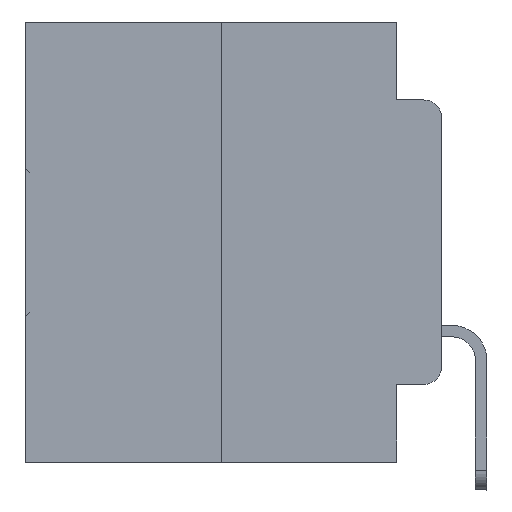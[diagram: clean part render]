
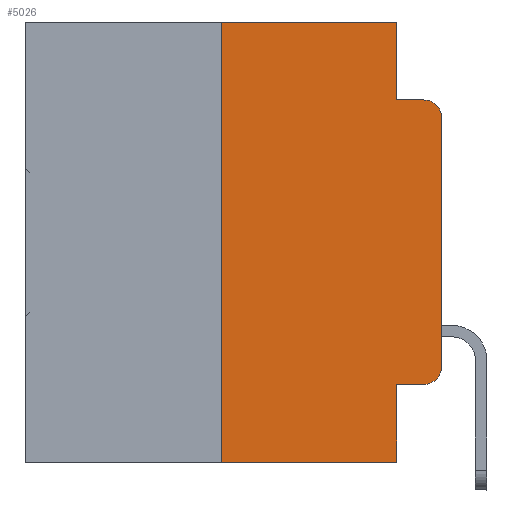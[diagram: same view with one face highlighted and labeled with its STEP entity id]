
A CAD part, left-side view. The second image highlights one B-rep face of the part: STEP entity #5026.
In plain terms, the highlighted planar face has unit normal (-1, 0, 0).
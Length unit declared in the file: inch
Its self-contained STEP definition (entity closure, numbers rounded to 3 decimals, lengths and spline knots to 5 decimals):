
#214 = ORIENTED_EDGE ( 'NONE', *, *, #19649, .F. ) ;
#864 = VERTEX_POINT ( 'NONE', #28707 ) ;
#908 = CARTESIAN_POINT ( 'NONE',  ( 0., 0.473, 0. ) ) ;
#1115 = DIRECTION ( 'NONE',  ( 1., 0., 0. ) ) ;
#1442 = ORIENTED_EDGE ( 'NONE', *, *, #26857, .F. ) ;
#1703 = LINE ( 'NONE', #908, #13015 ) ;
#1744 = DIRECTION ( 'NONE',  ( 0., 0., -1. ) ) ;
#2532 = VERTEX_POINT ( 'NONE', #3071 ) ;
#2735 = ORIENTED_EDGE ( 'NONE', *, *, #4568, .T. ) ;
#2929 = LINE ( 'NONE', #17786, #11492 ) ;
#3071 = CARTESIAN_POINT ( 'NONE',  ( 0., 0., -0.3915 ) ) ;
#3426 = ORIENTED_EDGE ( 'NONE', *, *, #12831, .T. ) ;
#3738 = DIRECTION ( 'NONE',  ( 0., -1., 0. ) ) ;
#3915 = VERTEX_POINT ( 'NONE', #12719 ) ;
#4088 = EDGE_CURVE ( 'NONE', #23201, #19139, #2929, .T. ) ;
#4233 = CARTESIAN_POINT ( 'NONE',  ( 0., 0.02, -0.3915 ) ) ;
#4366 = LINE ( 'NONE', #6525, #6291 ) ;
#4568 = EDGE_CURVE ( 'NONE', #14420, #16784, #14978, .T. ) ;
#4625 = DIRECTION ( 'NONE',  ( 0., 0., 1. ) ) ;
#4961 = EDGE_CURVE ( 'NONE', #18920, #27669, #1703, .T. ) ;
#5026 = ADVANCED_FACE ( 'NONE', ( #26962 ), #18706, .F. ) ;
#5320 = CIRCLE ( 'NONE', #6911, 0.02 ) ;
#5344 = VECTOR ( 'NONE', #4625, 39.37008 ) ;
#5829 = DIRECTION ( 'NONE',  ( 0., 0., -1. ) ) ;
#6291 = VECTOR ( 'NONE', #1744, 39.37008 ) ;
#6369 = AXIS2_PLACEMENT_3D ( 'NONE', #25749, #1115, #18502 ) ;
#6510 = CARTESIAN_POINT ( 'NONE',  ( 0., 0.25, -0.5 ) ) ;
#6525 = CARTESIAN_POINT ( 'NONE',  ( 0., 0.051, 0. ) ) ;
#6529 = CARTESIAN_POINT ( 'NONE',  ( 0., 0.25, 0. ) ) ;
#6729 = DIRECTION ( 'NONE',  ( 0., 0., -1. ) ) ;
#6879 = CARTESIAN_POINT ( 'NONE',  ( 0., 0., 0. ) ) ;
#6911 = AXIS2_PLACEMENT_3D ( 'NONE', #4233, #29305, #6729 ) ;
#6956 = CARTESIAN_POINT ( 'NONE',  ( 0., 0.051, -0.5 ) ) ;
#7088 = ORIENTED_EDGE ( 'NONE', *, *, #9439, .T. ) ;
#7480 = LINE ( 'NONE', #6879, #28429 ) ;
#7897 = VECTOR ( 'NONE', #25131, 39.37008 ) ;
#8065 = CARTESIAN_POINT ( 'NONE',  ( 0., 0.473, -0.5 ) ) ;
#8171 = DIRECTION ( 'NONE',  ( 0., -1., 0. ) ) ;
#8917 = CARTESIAN_POINT ( 'NONE',  ( 0., 0., -0.1085 ) ) ;
#9439 = EDGE_CURVE ( 'NONE', #864, #2532, #5320, .T. ) ;
#9491 = ORIENTED_EDGE ( 'NONE', *, *, #23891, .F. ) ;
#9516 = ORIENTED_EDGE ( 'NONE', *, *, #18030, .T. ) ;
#9901 = ORIENTED_EDGE ( 'NONE', *, *, #23281, .T. ) ;
#11492 = VECTOR ( 'NONE', #5829, 39.37008 ) ;
#11805 = DIRECTION ( 'NONE',  ( 0., 0., 1. ) ) ;
#12719 = CARTESIAN_POINT ( 'NONE',  ( 0., 0.051, -0.0885 ) ) ;
#12831 = EDGE_CURVE ( 'NONE', #27946, #19139, #21442, .T. ) ;
#13015 = VECTOR ( 'NONE', #3738, 39.37008 ) ;
#14321 = DIRECTION ( 'NONE',  ( 0., 0., -1. ) ) ;
#14345 = CARTESIAN_POINT ( 'NONE',  ( 0., 0.051, -0.0885 ) ) ;
#14387 = CARTESIAN_POINT ( 'NONE',  ( 0., 0.051, -0.4115 ) ) ;
#14420 = VERTEX_POINT ( 'NONE', #8917 ) ;
#14978 = CIRCLE ( 'NONE', #28000, 0.02 ) ;
#16452 = ORIENTED_EDGE ( 'NONE', *, *, #4961, .F. ) ;
#16784 = VERTEX_POINT ( 'NONE', #21985 ) ;
#17171 = VECTOR ( 'NONE', #22247, 39.37008 ) ;
#17187 = VECTOR ( 'NONE', #8171, 39.37008 ) ;
#17786 = CARTESIAN_POINT ( 'NONE',  ( 0., 0.051, 0. ) ) ;
#17868 = CARTESIAN_POINT ( 'NONE',  ( 0., 0.051, -0.4115 ) ) ;
#18030 = EDGE_CURVE ( 'NONE', #23201, #864, #28075, .T. ) ;
#18502 = DIRECTION ( 'NONE',  ( 0., 0., -1. ) ) ;
#18706 = PLANE ( 'NONE',  #6369 ) ;
#18715 = ORIENTED_EDGE ( 'NONE', *, *, #4088, .F. ) ;
#18920 = VERTEX_POINT ( 'NONE', #6529 ) ;
#19139 = VERTEX_POINT ( 'NONE', #6956 ) ;
#19496 = CARTESIAN_POINT ( 'NONE',  ( 0., 0.25, 0. ) ) ;
#19649 = EDGE_CURVE ( 'NONE', #3915, #16784, #24896, .T. ) ;
#21442 = LINE ( 'NONE', #8065, #17187 ) ;
#21985 = CARTESIAN_POINT ( 'NONE',  ( 0., 0.02, -0.0885 ) ) ;
#22247 = DIRECTION ( 'NONE',  ( 0., -1., 0. ) ) ;
#23201 = VERTEX_POINT ( 'NONE', #14387 ) ;
#23281 = EDGE_CURVE ( 'NONE', #2532, #14420, #7480, .T. ) ;
#23891 = EDGE_CURVE ( 'NONE', #27669, #3915, #4366, .T. ) ;
#24471 = DIRECTION ( 'NONE',  ( -1., 0., 0. ) ) ;
#24896 = LINE ( 'NONE', #14345, #17171 ) ;
#25131 = DIRECTION ( 'NONE',  ( 0., -1., 0. ) ) ;
#25749 = CARTESIAN_POINT ( 'NONE',  ( 0., 0.473, 0. ) ) ;
#26857 = EDGE_CURVE ( 'NONE', #27946, #18920, #29039, .T. ) ;
#26871 = CARTESIAN_POINT ( 'NONE',  ( 0., 0.02, -0.1085 ) ) ;
#26962 = FACE_OUTER_BOUND ( 'NONE', #29751, .T. ) ;
#27669 = VERTEX_POINT ( 'NONE', #27696 ) ;
#27696 = CARTESIAN_POINT ( 'NONE',  ( 0., 0.051, 0. ) ) ;
#27946 = VERTEX_POINT ( 'NONE', #6510 ) ;
#28000 = AXIS2_PLACEMENT_3D ( 'NONE', #26871, #24471, #14321 ) ;
#28075 = LINE ( 'NONE', #17868, #7897 ) ;
#28429 = VECTOR ( 'NONE', #11805, 39.37008 ) ;
#28707 = CARTESIAN_POINT ( 'NONE',  ( 0., 0.02, -0.4115 ) ) ;
#29039 = LINE ( 'NONE', #19496, #5344 ) ;
#29305 = DIRECTION ( 'NONE',  ( -1., 0., 0. ) ) ;
#29751 = EDGE_LOOP ( 'NONE', ( #9901, #2735, #214, #9491, #16452, #1442, #3426, #18715, #9516, #7088 ) ) ;
